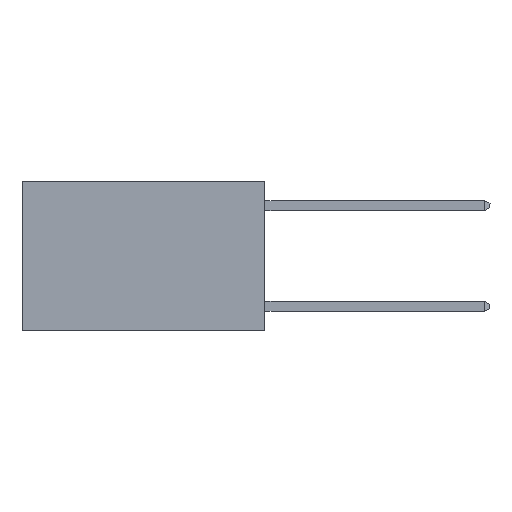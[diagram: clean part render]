
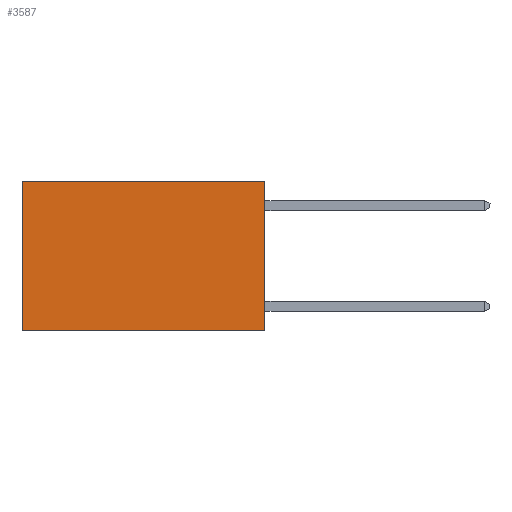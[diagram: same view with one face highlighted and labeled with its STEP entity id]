
A CAD part, left-side view. The second image highlights one B-rep face of the part: STEP entity #3587.
In plain terms, the highlighted planar face has unit normal (-1, 0, 0).
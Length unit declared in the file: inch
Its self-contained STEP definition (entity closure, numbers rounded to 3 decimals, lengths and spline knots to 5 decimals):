
#289 = FACE_OUTER_BOUND ( 'NONE', #6725, .T. ) ;
#319 = DIRECTION ( 'NONE',  ( 0., 0., -1. ) ) ;
#411 = CARTESIAN_POINT ( 'NONE',  ( 0.2625, 0., -0.37 ) ) ;
#864 = LINE ( 'NONE', #6782, #2859 ) ;
#2018 = VECTOR ( 'NONE', #3919, 39.37008 ) ;
#2224 = ORIENTED_EDGE ( 'NONE', *, *, #5137, .T. ) ;
#2342 = ORIENTED_EDGE ( 'NONE', *, *, #7618, .F. ) ;
#2423 = CARTESIAN_POINT ( 'NONE',  ( 0.2625, 0., -0.37 ) ) ;
#2666 = EDGE_CURVE ( 'NONE', #4153, #2900, #5980, .T. ) ;
#2670 = DIRECTION ( 'NONE',  ( 0., 1., 0. ) ) ;
#2813 = VERTEX_POINT ( 'NONE', #2423 ) ;
#2859 = VECTOR ( 'NONE', #7481, 39.37008 ) ;
#2900 = VERTEX_POINT ( 'NONE', #5512 ) ;
#3587 = ADVANCED_FACE ( 'NONE', ( #289 ), #4044, .F. ) ;
#3818 = CARTESIAN_POINT ( 'NONE',  ( 0.2625, 0.6, 0. ) ) ;
#3886 = CARTESIAN_POINT ( 'NONE',  ( 0.2625, 0., 0. ) ) ;
#3919 = DIRECTION ( 'NONE',  ( 0., 1., 0. ) ) ;
#4008 = LINE ( 'NONE', #3886, #2018 ) ;
#4044 = PLANE ( 'NONE',  #5344 ) ;
#4121 = VERTEX_POINT ( 'NONE', #4672 ) ;
#4153 = VERTEX_POINT ( 'NONE', #8383 ) ;
#4324 = VECTOR ( 'NONE', #2670, 39.37008 ) ;
#4672 = CARTESIAN_POINT ( 'NONE',  ( 0.2625, 0., 0. ) ) ;
#4771 = DIRECTION ( 'NONE',  ( 1., 0., 0. ) ) ;
#5137 = EDGE_CURVE ( 'NONE', #4121, #4153, #4008, .T. ) ;
#5344 = AXIS2_PLACEMENT_3D ( 'NONE', #9154, #4771, #319 ) ;
#5512 = CARTESIAN_POINT ( 'NONE',  ( 0.2625, 0.6, -0.37 ) ) ;
#5980 = LINE ( 'NONE', #3818, #7701 ) ;
#6269 = LINE ( 'NONE', #411, #4324 ) ;
#6682 = EDGE_CURVE ( 'NONE', #2813, #2900, #6269, .T. ) ;
#6725 = EDGE_LOOP ( 'NONE', ( #8213, #9037, #2342, #2224 ) ) ;
#6782 = CARTESIAN_POINT ( 'NONE',  ( 0.2625, 0., 0. ) ) ;
#7481 = DIRECTION ( 'NONE',  ( 0., 0., -1. ) ) ;
#7618 = EDGE_CURVE ( 'NONE', #4121, #2813, #864, .T. ) ;
#7701 = VECTOR ( 'NONE', #8184, 39.37008 ) ;
#8184 = DIRECTION ( 'NONE',  ( 0., 0., -1. ) ) ;
#8213 = ORIENTED_EDGE ( 'NONE', *, *, #2666, .T. ) ;
#8383 = CARTESIAN_POINT ( 'NONE',  ( 0.2625, 0.6, 0. ) ) ;
#9037 = ORIENTED_EDGE ( 'NONE', *, *, #6682, .F. ) ;
#9154 = CARTESIAN_POINT ( 'NONE',  ( 0.2625, 0., 0. ) ) ;
